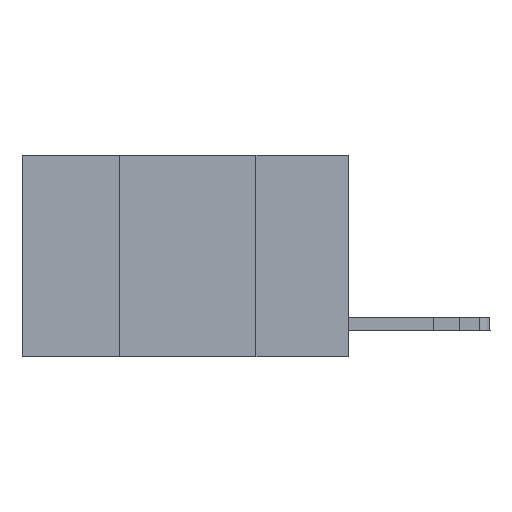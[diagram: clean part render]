
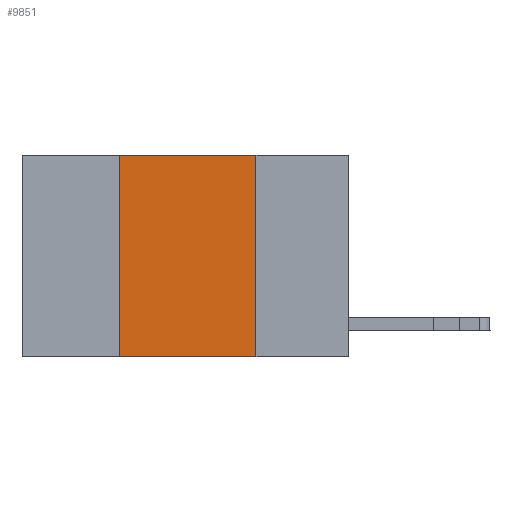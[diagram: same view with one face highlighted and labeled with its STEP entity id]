
A CAD part, left-side view. The second image highlights one B-rep face of the part: STEP entity #9851.
In plain terms, the highlighted planar face has unit normal (-1, 0, 0).
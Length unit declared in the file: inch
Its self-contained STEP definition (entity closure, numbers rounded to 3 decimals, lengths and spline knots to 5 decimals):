
#1470 = CARTESIAN_POINT ( 'NONE',  ( 0., 0.17, -0.37 ) ) ;
#1827 = EDGE_CURVE ( 'NONE', #9709, #6248, #2830, .T. ) ;
#1989 = LINE ( 'NONE', #13025, #9138 ) ;
#2830 = LINE ( 'NONE', #5464, #11607 ) ;
#3947 = ORIENTED_EDGE ( 'NONE', *, *, #14677, .F. ) ;
#4427 = CARTESIAN_POINT ( 'NONE',  ( 0., 0.6, 0. ) ) ;
#4512 = DIRECTION ( 'NONE',  ( 0., 0., -1. ) ) ;
#5324 = AXIS2_PLACEMENT_3D ( 'NONE', #4427, #8362, #4512 ) ;
#5464 = CARTESIAN_POINT ( 'NONE',  ( 0., 0.6, -0.37 ) ) ;
#6129 = LINE ( 'NONE', #10305, #17235 ) ;
#6248 = VERTEX_POINT ( 'NONE', #1470 ) ;
#7685 = CARTESIAN_POINT ( 'NONE',  ( 0., 0.6, 0. ) ) ;
#7730 = VECTOR ( 'NONE', #10216, 39.37008 ) ;
#8002 = DIRECTION ( 'NONE',  ( 0., -1., 0. ) ) ;
#8362 = DIRECTION ( 'NONE',  ( 1., 0., 0. ) ) ;
#9074 = FACE_OUTER_BOUND ( 'NONE', #14019, .T. ) ;
#9138 = VECTOR ( 'NONE', #9941, 39.37008 ) ;
#9499 = PLANE ( 'NONE',  #5324 ) ;
#9709 = VERTEX_POINT ( 'NONE', #15846 ) ;
#9851 = ADVANCED_FACE ( 'NONE', ( #9074 ), #9499, .F. ) ;
#9941 = DIRECTION ( 'NONE',  ( 0., 0., 1. ) ) ;
#10132 = ORIENTED_EDGE ( 'NONE', *, *, #12731, .F. ) ;
#10216 = DIRECTION ( 'NONE',  ( 0., -1., 0. ) ) ;
#10305 = CARTESIAN_POINT ( 'NONE',  ( 0., 0.17, 0. ) ) ;
#11354 = DIRECTION ( 'NONE',  ( 0., 0., -1. ) ) ;
#11425 = ORIENTED_EDGE ( 'NONE', *, *, #1827, .T. ) ;
#11607 = VECTOR ( 'NONE', #8002, 39.37008 ) ;
#12731 = EDGE_CURVE ( 'NONE', #13690, #13681, #16980, .T. ) ;
#13025 = CARTESIAN_POINT ( 'NONE',  ( 0., 0.42, 0. ) ) ;
#13681 = VERTEX_POINT ( 'NONE', #16188 ) ;
#13690 = VERTEX_POINT ( 'NONE', #14768 ) ;
#14019 = EDGE_LOOP ( 'NONE', ( #3947, #10132, #14775, #11425 ) ) ;
#14677 = EDGE_CURVE ( 'NONE', #13681, #6248, #6129, .T. ) ;
#14698 = EDGE_CURVE ( 'NONE', #9709, #13690, #1989, .T. ) ;
#14768 = CARTESIAN_POINT ( 'NONE',  ( 0., 0.42, 0. ) ) ;
#14775 = ORIENTED_EDGE ( 'NONE', *, *, #14698, .F. ) ;
#15846 = CARTESIAN_POINT ( 'NONE',  ( 0., 0.42, -0.37 ) ) ;
#16188 = CARTESIAN_POINT ( 'NONE',  ( 0., 0.17, 0. ) ) ;
#16980 = LINE ( 'NONE', #7685, #7730 ) ;
#17235 = VECTOR ( 'NONE', #11354, 39.37008 ) ;
